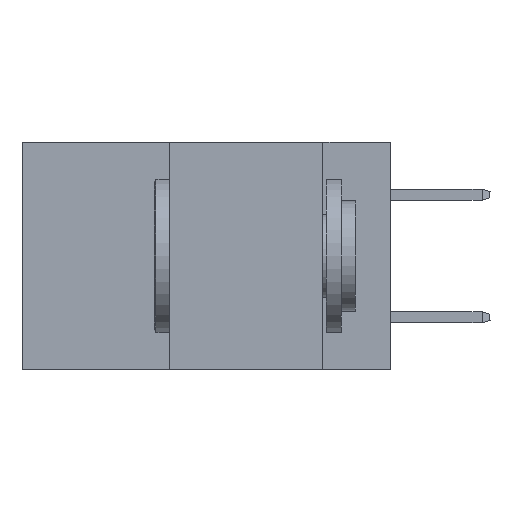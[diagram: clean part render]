
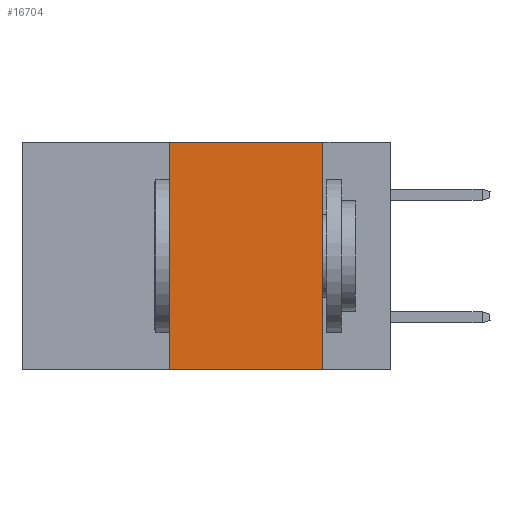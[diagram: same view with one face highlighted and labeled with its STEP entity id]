
A CAD part, left-side view. The second image highlights one B-rep face of the part: STEP entity #16704.
In plain terms, the highlighted planar face has unit normal (-1, 0, 0).
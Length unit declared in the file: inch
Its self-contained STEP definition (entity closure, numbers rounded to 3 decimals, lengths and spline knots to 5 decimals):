
#16 = ORIENTED_EDGE ( 'NONE', *, *, #18645, .F. ) ;
#2100 = VERTEX_POINT ( 'NONE', #18804 ) ;
#2421 = EDGE_LOOP ( 'NONE', ( #3550, #4817, #16, #10635 ) ) ;
#3466 = CARTESIAN_POINT ( 'NONE',  ( 0., 0.6, 0. ) ) ;
#3550 = ORIENTED_EDGE ( 'NONE', *, *, #16381, .F. ) ;
#3935 = LINE ( 'NONE', #19949, #23420 ) ;
#4817 = ORIENTED_EDGE ( 'NONE', *, *, #22010, .F. ) ;
#6852 = DIRECTION ( 'NONE',  ( 0., -1., 0. ) ) ;
#7995 = CARTESIAN_POINT ( 'NONE',  ( 0., 0.11, 0. ) ) ;
#9564 = LINE ( 'NONE', #3466, #18851 ) ;
#9906 = DIRECTION ( 'NONE',  ( 0., 0., -1. ) ) ;
#10491 = CARTESIAN_POINT ( 'NONE',  ( 0., 0.36, 0. ) ) ;
#10635 = ORIENTED_EDGE ( 'NONE', *, *, #22656, .T. ) ;
#11241 = CARTESIAN_POINT ( 'NONE',  ( 0., 0.36, -0.37 ) ) ;
#11287 = CARTESIAN_POINT ( 'NONE',  ( 0., 0.6, 0. ) ) ;
#11934 = VECTOR ( 'NONE', #9906, 39.37008 ) ;
#12222 = VERTEX_POINT ( 'NONE', #11241 ) ;
#12509 = LINE ( 'NONE', #19055, #11934 ) ;
#13190 = DIRECTION ( 'NONE',  ( 0., 0., -1. ) ) ;
#13688 = FACE_OUTER_BOUND ( 'NONE', #2421, .T. ) ;
#14720 = LINE ( 'NONE', #22172, #23914 ) ;
#14732 = VERTEX_POINT ( 'NONE', #10491 ) ;
#16381 = EDGE_CURVE ( 'NONE', #24171, #2100, #12509, .T. ) ;
#16499 = AXIS2_PLACEMENT_3D ( 'NONE', #11287, #24189, #13190 ) ;
#16704 = ADVANCED_FACE ( 'NONE', ( #13688 ), #22339, .F. ) ;
#16960 = DIRECTION ( 'NONE',  ( 0., -1., 0. ) ) ;
#18645 = EDGE_CURVE ( 'NONE', #12222, #14732, #14720, .T. ) ;
#18804 = CARTESIAN_POINT ( 'NONE',  ( 0., 0.11, -0.37 ) ) ;
#18851 = VECTOR ( 'NONE', #16960, 39.37008 ) ;
#19055 = CARTESIAN_POINT ( 'NONE',  ( 0., 0.11, 0. ) ) ;
#19949 = CARTESIAN_POINT ( 'NONE',  ( 0., 0.6, -0.37 ) ) ;
#22010 = EDGE_CURVE ( 'NONE', #14732, #24171, #9564, .T. ) ;
#22172 = CARTESIAN_POINT ( 'NONE',  ( 0., 0.36, 0. ) ) ;
#22339 = PLANE ( 'NONE',  #16499 ) ;
#22656 = EDGE_CURVE ( 'NONE', #12222, #2100, #3935, .T. ) ;
#23420 = VECTOR ( 'NONE', #6852, 39.37008 ) ;
#23914 = VECTOR ( 'NONE', #24027, 39.37008 ) ;
#24027 = DIRECTION ( 'NONE',  ( 0., 0., 1. ) ) ;
#24171 = VERTEX_POINT ( 'NONE', #7995 ) ;
#24189 = DIRECTION ( 'NONE',  ( 1., 0., 0. ) ) ;
